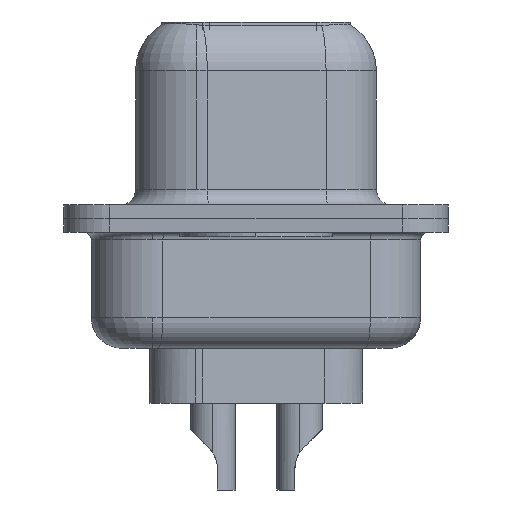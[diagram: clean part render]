
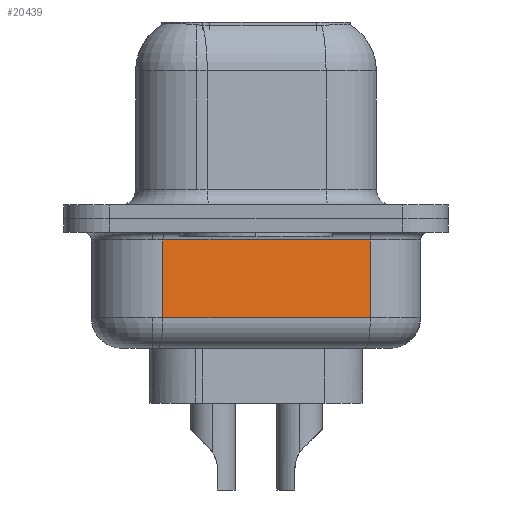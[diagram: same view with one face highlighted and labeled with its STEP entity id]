
A CAD part, left-side view. The second image highlights one B-rep face of the part: STEP entity #20439.
In plain terms, the highlighted planar face has unit normal (-0.985, -0.174, 0).
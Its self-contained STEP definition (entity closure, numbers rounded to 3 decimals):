
#173 = DIRECTION ( 'NONE',  ( 0., 0., 1. ) ) ;
#254 = DIRECTION ( 'NONE',  ( 0., 0., 1. ) ) ;
#413 = LINE ( 'NONE', #9764, #10784 ) ;
#812 = EDGE_CURVE ( 'NONE', #9360, #17879, #16540, .T. ) ;
#981 = PLANE ( 'NONE',  #16644 ) ;
#1632 = EDGE_CURVE ( 'NONE', #17545, #5432, #413, .T. ) ;
#3232 = CARTESIAN_POINT ( 'NONE',  ( 2.85, 3.053, -3.25 ) ) ;
#3739 = ORIENTED_EDGE ( 'NONE', *, *, #812, .T. ) ;
#3959 = EDGE_CURVE ( 'NONE', #17879, #5432, #4668, .T. ) ;
#4668 = LINE ( 'NONE', #22970, #5220 ) ;
#4933 = FACE_OUTER_BOUND ( 'NONE', #20571, .T. ) ;
#5220 = VECTOR ( 'NONE', #11987, 1000. ) ;
#5432 = VERTEX_POINT ( 'NONE', #19169 ) ;
#6125 = VECTOR ( 'NONE', #17995, 1000. ) ;
#6914 = CARTESIAN_POINT ( 'NONE',  ( 2.85, 3.053, -3.25 ) ) ;
#8521 = CARTESIAN_POINT ( 'NONE',  ( 2.85, 3.053, -4.25 ) ) ;
#8688 = EDGE_CURVE ( 'NONE', #17545, #9360, #19916, .T. ) ;
#9360 = VERTEX_POINT ( 'NONE', #10034 ) ;
#9764 = CARTESIAN_POINT ( 'NONE',  ( 2.85, 3.053, -4.25 ) ) ;
#10034 = CARTESIAN_POINT ( 'NONE',  ( 4.049, -3.747, -3.25 ) ) ;
#10784 = VECTOR ( 'NONE', #173, 1000. ) ;
#11987 = DIRECTION ( 'NONE',  ( -0.174, 0.985, 0. ) ) ;
#12739 = VECTOR ( 'NONE', #254, 1000. ) ;
#15830 = DIRECTION ( 'NONE',  ( 0.985, 0.174, 0. ) ) ;
#16015 = CARTESIAN_POINT ( 'NONE',  ( 4.049, -3.747, -0.7 ) ) ;
#16540 = LINE ( 'NONE', #16653, #12739 ) ;
#16644 = AXIS2_PLACEMENT_3D ( 'NONE', #8521, #15830, #17484 ) ;
#16653 = CARTESIAN_POINT ( 'NONE',  ( 4.049, -3.747, -4.25 ) ) ;
#16848 = ORIENTED_EDGE ( 'NONE', *, *, #1632, .F. ) ;
#17484 = DIRECTION ( 'NONE',  ( -0.174, 0.985, 0. ) ) ;
#17545 = VERTEX_POINT ( 'NONE', #3232 ) ;
#17684 = ORIENTED_EDGE ( 'NONE', *, *, #3959, .T. ) ;
#17879 = VERTEX_POINT ( 'NONE', #16015 ) ;
#17995 = DIRECTION ( 'NONE',  ( 0.174, -0.985, 0. ) ) ;
#19169 = CARTESIAN_POINT ( 'NONE',  ( 2.85, 3.053, -0.7 ) ) ;
#19669 = ORIENTED_EDGE ( 'NONE', *, *, #8688, .T. ) ;
#19916 = LINE ( 'NONE', #6914, #6125 ) ;
#20439 = ADVANCED_FACE ( 'NONE', ( #4933 ), #981, .F. ) ;
#20571 = EDGE_LOOP ( 'NONE', ( #16848, #19669, #3739, #17684 ) ) ;
#22970 = CARTESIAN_POINT ( 'NONE',  ( 2.85, 3.053, -0.7 ) ) ;
